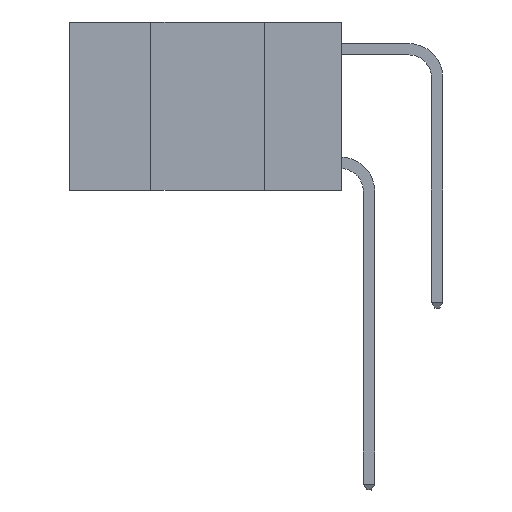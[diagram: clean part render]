
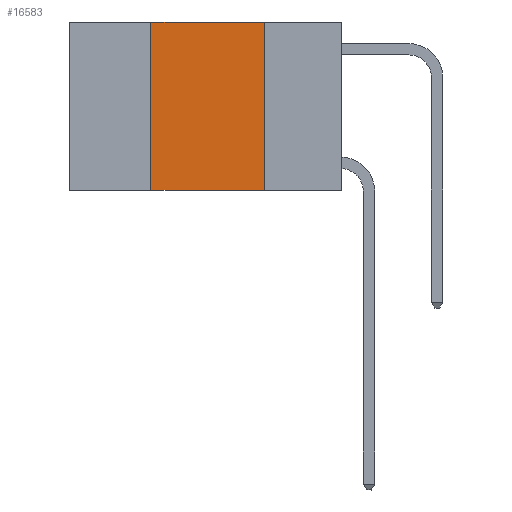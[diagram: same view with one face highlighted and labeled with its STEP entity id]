
A CAD part, left-side view. The second image highlights one B-rep face of the part: STEP entity #16583.
In plain terms, the highlighted planar face has unit normal (-1, 0, 0).
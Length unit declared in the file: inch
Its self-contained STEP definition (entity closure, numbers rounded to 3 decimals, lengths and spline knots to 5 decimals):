
#4 = DIRECTION ( 'NONE',  ( 0., 0., -1. ) ) ;
#867 = VECTOR ( 'NONE', #4, 39.37008 ) ;
#1209 = PLANE ( 'NONE',  #19646 ) ;
#1628 = DIRECTION ( 'NONE',  ( 0., 0., -1. ) ) ;
#1828 = CARTESIAN_POINT ( 'NONE',  ( 0., 0.17, -0.37 ) ) ;
#2467 = DIRECTION ( 'NONE',  ( 0., -1., 0. ) ) ;
#2596 = LINE ( 'NONE', #16474, #12960 ) ;
#3500 = VECTOR ( 'NONE', #8469, 39.37008 ) ;
#4771 = CARTESIAN_POINT ( 'NONE',  ( 0., 0.6, -0.37 ) ) ;
#4981 = VERTEX_POINT ( 'NONE', #8840 ) ;
#5148 = LINE ( 'NONE', #12904, #867 ) ;
#6173 = ORIENTED_EDGE ( 'NONE', *, *, #12709, .F. ) ;
#8414 = LINE ( 'NONE', #4771, #3500 ) ;
#8469 = DIRECTION ( 'NONE',  ( 0., -1., 0. ) ) ;
#8524 = EDGE_LOOP ( 'NONE', ( #9943, #6173, #11676, #12270 ) ) ;
#8840 = CARTESIAN_POINT ( 'NONE',  ( 0., 0.42, -0.37 ) ) ;
#9382 = EDGE_CURVE ( 'NONE', #4981, #15521, #8414, .T. ) ;
#9943 = ORIENTED_EDGE ( 'NONE', *, *, #20798, .F. ) ;
#11079 = EDGE_CURVE ( 'NONE', #4981, #11517, #2596, .T. ) ;
#11517 = VERTEX_POINT ( 'NONE', #15813 ) ;
#11634 = CARTESIAN_POINT ( 'NONE',  ( 0., 0.6, 0. ) ) ;
#11676 = ORIENTED_EDGE ( 'NONE', *, *, #11079, .F. ) ;
#12270 = ORIENTED_EDGE ( 'NONE', *, *, #9382, .T. ) ;
#12634 = DIRECTION ( 'NONE',  ( 1., 0., 0. ) ) ;
#12709 = EDGE_CURVE ( 'NONE', #11517, #17040, #18944, .T. ) ;
#12904 = CARTESIAN_POINT ( 'NONE',  ( 0., 0.17, 0. ) ) ;
#12960 = VECTOR ( 'NONE', #14616, 39.37008 ) ;
#13875 = CARTESIAN_POINT ( 'NONE',  ( 0., 0.17, 0. ) ) ;
#14616 = DIRECTION ( 'NONE',  ( 0., 0., 1. ) ) ;
#15521 = VERTEX_POINT ( 'NONE', #1828 ) ;
#15813 = CARTESIAN_POINT ( 'NONE',  ( 0., 0.42, 0. ) ) ;
#16474 = CARTESIAN_POINT ( 'NONE',  ( 0., 0.42, 0. ) ) ;
#16583 = ADVANCED_FACE ( 'NONE', ( #17335 ), #1209, .F. ) ;
#17040 = VERTEX_POINT ( 'NONE', #13875 ) ;
#17335 = FACE_OUTER_BOUND ( 'NONE', #8524, .T. ) ;
#18371 = VECTOR ( 'NONE', #2467, 39.37008 ) ;
#18944 = LINE ( 'NONE', #11634, #18371 ) ;
#19646 = AXIS2_PLACEMENT_3D ( 'NONE', #19847, #12634, #1628 ) ;
#19847 = CARTESIAN_POINT ( 'NONE',  ( 0., 0.6, 0. ) ) ;
#20798 = EDGE_CURVE ( 'NONE', #17040, #15521, #5148, .T. ) ;
